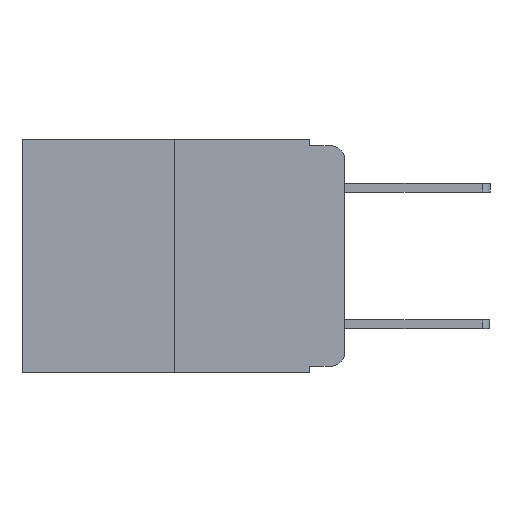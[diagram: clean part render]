
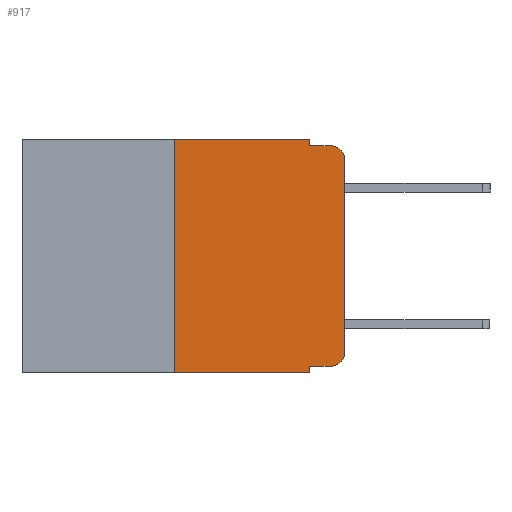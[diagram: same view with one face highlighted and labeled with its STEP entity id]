
A CAD part, left-side view. The second image highlights one B-rep face of the part: STEP entity #917.
In plain terms, the highlighted planar face has unit normal (-1, 0, 0).
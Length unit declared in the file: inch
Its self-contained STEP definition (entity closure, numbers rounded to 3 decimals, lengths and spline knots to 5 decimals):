
#183 = CIRCLE ( 'NONE', #7857, 0.02 ) ;
#425 = CARTESIAN_POINT ( 'NONE',  ( 0., 0.02, -0.333 ) ) ;
#459 = DIRECTION ( 'NONE',  ( -1., 0., 0. ) ) ;
#479 = CARTESIAN_POINT ( 'NONE',  ( 0., 0.051, -0.01 ) ) ;
#496 = CARTESIAN_POINT ( 'NONE',  ( 0., 0.051, -0.343 ) ) ;
#656 = DIRECTION ( 'NONE',  ( 0., 0., -1. ) ) ;
#740 = ORIENTED_EDGE ( 'NONE', *, *, #13363, .F. ) ;
#917 = ADVANCED_FACE ( 'NONE', ( #11313 ), #1652, .F. ) ;
#973 = CARTESIAN_POINT ( 'NONE',  ( 0., 0.473, -0.343 ) ) ;
#1041 = LINE ( 'NONE', #13357, #12726 ) ;
#1203 = VECTOR ( 'NONE', #7888, 39.37008 ) ;
#1244 = DIRECTION ( 'NONE',  ( 0., -1., 0. ) ) ;
#1363 = EDGE_CURVE ( 'NONE', #4186, #4727, #183, .T. ) ;
#1525 = DIRECTION ( 'NONE',  ( 1., 0., 0. ) ) ;
#1652 = PLANE ( 'NONE',  #11668 ) ;
#1969 = CARTESIAN_POINT ( 'NONE',  ( 0., 0.051, -0.333 ) ) ;
#2199 = EDGE_CURVE ( 'NONE', #6602, #4186, #1041, .T. ) ;
#2522 = ORIENTED_EDGE ( 'NONE', *, *, #12641, .F. ) ;
#2773 = VERTEX_POINT ( 'NONE', #10263 ) ;
#2788 = LINE ( 'NONE', #9711, #11130 ) ;
#2901 = ORIENTED_EDGE ( 'NONE', *, *, #14037, .F. ) ;
#2955 = VECTOR ( 'NONE', #5394, 39.37008 ) ;
#2987 = CARTESIAN_POINT ( 'NONE',  ( 0., 0., -0.03 ) ) ;
#3006 = VECTOR ( 'NONE', #3182, 39.37008 ) ;
#3105 = VECTOR ( 'NONE', #5422, 39.37008 ) ;
#3182 = DIRECTION ( 'NONE',  ( 0., -1., 0. ) ) ;
#3546 = ORIENTED_EDGE ( 'NONE', *, *, #10645, .F. ) ;
#3709 = ORIENTED_EDGE ( 'NONE', *, *, #10545, .T. ) ;
#4186 = VERTEX_POINT ( 'NONE', #2987 ) ;
#4283 = CARTESIAN_POINT ( 'NONE',  ( 0., 0.02, -0.03 ) ) ;
#4727 = VERTEX_POINT ( 'NONE', #13616 ) ;
#4753 = VERTEX_POINT ( 'NONE', #425 ) ;
#4792 = ORIENTED_EDGE ( 'NONE', *, *, #2199, .T. ) ;
#4868 = CARTESIAN_POINT ( 'NONE',  ( 0., 0., -0.313 ) ) ;
#5034 = ORIENTED_EDGE ( 'NONE', *, *, #11261, .T. ) ;
#5392 = CARTESIAN_POINT ( 'NONE',  ( 0., 0.473, 0. ) ) ;
#5394 = DIRECTION ( 'NONE',  ( 0., 0., 1. ) ) ;
#5422 = DIRECTION ( 'NONE',  ( 0., 0., -1. ) ) ;
#6017 = CIRCLE ( 'NONE', #6369, 0.02 ) ;
#6113 = CARTESIAN_POINT ( 'NONE',  ( 0., 0.473, 0. ) ) ;
#6114 = LINE ( 'NONE', #8662, #3105 ) ;
#6253 = CARTESIAN_POINT ( 'NONE',  ( 0., 0.051, 0. ) ) ;
#6369 = AXIS2_PLACEMENT_3D ( 'NONE', #7485, #459, #8542 ) ;
#6485 = DIRECTION ( 'NONE',  ( 0., -1., 0. ) ) ;
#6602 = VERTEX_POINT ( 'NONE', #4868 ) ;
#7008 = LINE ( 'NONE', #973, #1203 ) ;
#7485 = CARTESIAN_POINT ( 'NONE',  ( 0., 0.02, -0.313 ) ) ;
#7737 = CARTESIAN_POINT ( 'NONE',  ( 0., 0.051, -0.333 ) ) ;
#7857 = AXIS2_PLACEMENT_3D ( 'NONE', #4283, #10894, #10952 ) ;
#7888 = DIRECTION ( 'NONE',  ( 0., -1., 0. ) ) ;
#7918 = LINE ( 'NONE', #5392, #13117 ) ;
#8108 = CARTESIAN_POINT ( 'NONE',  ( 0., 0.051, -0.01 ) ) ;
#8492 = VECTOR ( 'NONE', #1244, 39.37008 ) ;
#8527 = CARTESIAN_POINT ( 'NONE',  ( 0., 0.25, 0. ) ) ;
#8538 = EDGE_LOOP ( 'NONE', ( #4792, #8630, #2901, #740, #3546, #2522, #14240, #12765, #5034, #3709 ) ) ;
#8542 = DIRECTION ( 'NONE',  ( 0., 0., -1. ) ) ;
#8630 = ORIENTED_EDGE ( 'NONE', *, *, #1363, .T. ) ;
#8662 = CARTESIAN_POINT ( 'NONE',  ( 0., 0.051, 0. ) ) ;
#8832 = VERTEX_POINT ( 'NONE', #496 ) ;
#9593 = VERTEX_POINT ( 'NONE', #479 ) ;
#9711 = CARTESIAN_POINT ( 'NONE',  ( 0., 0.051, 0. ) ) ;
#10188 = VERTEX_POINT ( 'NONE', #6253 ) ;
#10263 = CARTESIAN_POINT ( 'NONE',  ( 0., 0.25, -0.343 ) ) ;
#10545 = EDGE_CURVE ( 'NONE', #4753, #6602, #6017, .T. ) ;
#10645 = EDGE_CURVE ( 'NONE', #13257, #10188, #7918, .T. ) ;
#10894 = DIRECTION ( 'NONE',  ( -1., 0., 0. ) ) ;
#10952 = DIRECTION ( 'NONE',  ( 0., 0., -1. ) ) ;
#11130 = VECTOR ( 'NONE', #656, 39.37008 ) ;
#11261 = EDGE_CURVE ( 'NONE', #13834, #4753, #11788, .T. ) ;
#11313 = FACE_OUTER_BOUND ( 'NONE', #8538, .T. ) ;
#11668 = AXIS2_PLACEMENT_3D ( 'NONE', #6113, #1525, #12849 ) ;
#11788 = LINE ( 'NONE', #1969, #3006 ) ;
#11975 = EDGE_CURVE ( 'NONE', #13834, #8832, #2788, .T. ) ;
#12641 = EDGE_CURVE ( 'NONE', #2773, #13257, #14357, .T. ) ;
#12726 = VECTOR ( 'NONE', #12894, 39.37008 ) ;
#12765 = ORIENTED_EDGE ( 'NONE', *, *, #11975, .F. ) ;
#12849 = DIRECTION ( 'NONE',  ( 0., 0., -1. ) ) ;
#12894 = DIRECTION ( 'NONE',  ( 0., 0., 1. ) ) ;
#13117 = VECTOR ( 'NONE', #6485, 39.37008 ) ;
#13257 = VERTEX_POINT ( 'NONE', #8527 ) ;
#13357 = CARTESIAN_POINT ( 'NONE',  ( 0., 0., 0. ) ) ;
#13363 = EDGE_CURVE ( 'NONE', #10188, #9593, #6114, .T. ) ;
#13521 = EDGE_CURVE ( 'NONE', #2773, #8832, #7008, .T. ) ;
#13616 = CARTESIAN_POINT ( 'NONE',  ( 0., 0.02, -0.01 ) ) ;
#13823 = CARTESIAN_POINT ( 'NONE',  ( 0., 0.25, 0. ) ) ;
#13834 = VERTEX_POINT ( 'NONE', #7737 ) ;
#13991 = LINE ( 'NONE', #8108, #8492 ) ;
#14037 = EDGE_CURVE ( 'NONE', #9593, #4727, #13991, .T. ) ;
#14240 = ORIENTED_EDGE ( 'NONE', *, *, #13521, .T. ) ;
#14357 = LINE ( 'NONE', #13823, #2955 ) ;
